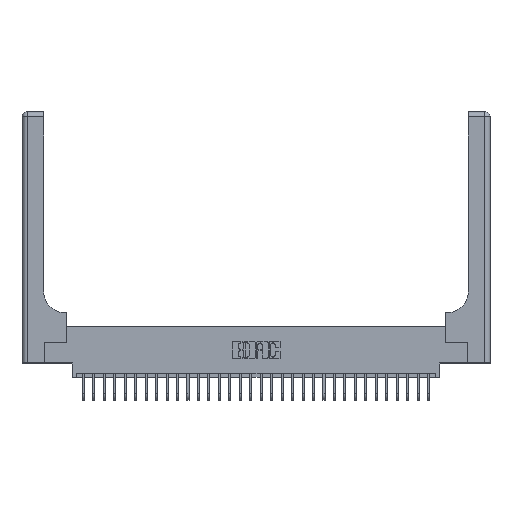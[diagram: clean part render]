
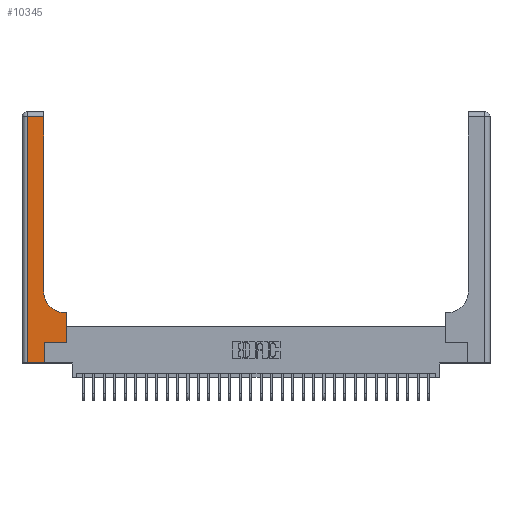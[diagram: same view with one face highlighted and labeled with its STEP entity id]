
A CAD part, top view. The second image highlights one B-rep face of the part: STEP entity #10345.
In plain terms, the highlighted planar face has unit normal (0, 0, 1).
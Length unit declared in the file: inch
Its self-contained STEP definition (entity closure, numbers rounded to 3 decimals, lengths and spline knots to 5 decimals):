
#349 = VECTOR ( 'NONE', #12767, 39.37008 ) ;
#1641 = VERTEX_POINT ( 'NONE', #20341 ) ;
#1968 = EDGE_CURVE ( 'NONE', #17609, #16469, #7856, .T. ) ;
#2002 = CIRCLE ( 'NONE', #9205, 0.25 ) ;
#2087 = LINE ( 'NONE', #19974, #28533 ) ;
#2182 = VERTEX_POINT ( 'NONE', #30388 ) ;
#2671 = LINE ( 'NONE', #3339, #16649 ) ;
#3339 = CARTESIAN_POINT ( 'NONE',  ( 0.265, 0.25, 0.37 ) ) ;
#3849 = VECTOR ( 'NONE', #8884, 39.37008 ) ;
#4074 = CARTESIAN_POINT ( 'NONE',  ( 0.528, 0.6, 0.37 ) ) ;
#4558 = LINE ( 'NONE', #20495, #28813 ) ;
#4676 = VERTEX_POINT ( 'NONE', #22473 ) ;
#5651 = CARTESIAN_POINT ( 'NONE',  ( 0.06, 3., 0.37 ) ) ;
#5925 = ORIENTED_EDGE ( 'NONE', *, *, #27238, .T. ) ;
#6271 = DIRECTION ( 'NONE',  ( -1., 0., 0. ) ) ;
#6275 = LINE ( 'NONE', #26719, #11770 ) ;
#6297 = CARTESIAN_POINT ( 'NONE',  ( 0.06, 2.94, 0.37 ) ) ;
#6916 = LINE ( 'NONE', #16647, #14210 ) ;
#7299 = VERTEX_POINT ( 'NONE', #15905 ) ;
#7306 = AXIS2_PLACEMENT_3D ( 'NONE', #10769, #20183, #6271 ) ;
#7359 = LINE ( 'NONE', #29495, #349 ) ;
#7856 = LINE ( 'NONE', #18640, #3849 ) ;
#8058 = CARTESIAN_POINT ( 'NONE',  ( 0.06, 0., 0.37 ) ) ;
#8654 = DIRECTION ( 'NONE',  ( 0., 1., 0. ) ) ;
#8852 = EDGE_LOOP ( 'NONE', ( #28516, #15959, #13714, #26668, #22316, #29290, #5925, #21931, #28116 ) ) ;
#8884 = DIRECTION ( 'NONE',  ( 1., 0., 0. ) ) ;
#8926 = EDGE_CURVE ( 'NONE', #4676, #24219, #2671, .T. ) ;
#9205 = AXIS2_PLACEMENT_3D ( 'NONE', #27649, #18677, #15988 ) ;
#9849 = VECTOR ( 'NONE', #25295, 39.37008 ) ;
#10345 = ADVANCED_FACE ( 'NONE', ( #15160 ), #22846, .F. ) ;
#10583 = DIRECTION ( 'NONE',  ( 0., 1., 0. ) ) ;
#10769 = CARTESIAN_POINT ( 'NONE',  ( 0., 3., 0.37 ) ) ;
#11770 = VECTOR ( 'NONE', #29083, 39.37008 ) ;
#12767 = DIRECTION ( 'NONE',  ( -1., 0., 0. ) ) ;
#13714 = ORIENTED_EDGE ( 'NONE', *, *, #15154, .T. ) ;
#14210 = VECTOR ( 'NONE', #16455, 39.37008 ) ;
#15139 = DIRECTION ( 'NONE',  ( 1., 0., 0. ) ) ;
#15154 = EDGE_CURVE ( 'NONE', #22289, #17609, #27829, .T. ) ;
#15160 = FACE_OUTER_BOUND ( 'NONE', #8852, .T. ) ;
#15905 = CARTESIAN_POINT ( 'NONE',  ( 0.26, 0.85, 0.37 ) ) ;
#15959 = ORIENTED_EDGE ( 'NONE', *, *, #23742, .T. ) ;
#15988 = DIRECTION ( 'NONE',  ( 1., 0., 0. ) ) ;
#16455 = DIRECTION ( 'NONE',  ( 0., 1., 0. ) ) ;
#16469 = VERTEX_POINT ( 'NONE', #17947 ) ;
#16647 = CARTESIAN_POINT ( 'NONE',  ( 0.528, 0.25, 0.37 ) ) ;
#16649 = VECTOR ( 'NONE', #15139, 39.37008 ) ;
#17053 = EDGE_CURVE ( 'NONE', #2182, #7299, #2002, .T. ) ;
#17589 = EDGE_CURVE ( 'NONE', #23135, #2182, #6275, .T. ) ;
#17609 = VERTEX_POINT ( 'NONE', #8058 ) ;
#17947 = CARTESIAN_POINT ( 'NONE',  ( 0.265, 0., 0.37 ) ) ;
#18640 = CARTESIAN_POINT ( 'NONE',  ( 0., 0., 0.37 ) ) ;
#18677 = DIRECTION ( 'NONE',  ( 0., 0., -1. ) ) ;
#19974 = CARTESIAN_POINT ( 'NONE',  ( 0.265, 0., 0.37 ) ) ;
#20183 = DIRECTION ( 'NONE',  ( 0., 0., -1. ) ) ;
#20341 = CARTESIAN_POINT ( 'NONE',  ( 0.26, 2.94, 0.37 ) ) ;
#20495 = CARTESIAN_POINT ( 'NONE',  ( 0.26, 3., 0.37 ) ) ;
#21931 = ORIENTED_EDGE ( 'NONE', *, *, #17589, .T. ) ;
#22289 = VERTEX_POINT ( 'NONE', #6297 ) ;
#22316 = ORIENTED_EDGE ( 'NONE', *, *, #27543, .T. ) ;
#22473 = CARTESIAN_POINT ( 'NONE',  ( 0.265, 0.25, 0.37 ) ) ;
#22846 = PLANE ( 'NONE',  #7306 ) ;
#23135 = VERTEX_POINT ( 'NONE', #4074 ) ;
#23742 = EDGE_CURVE ( 'NONE', #1641, #22289, #7359, .T. ) ;
#24219 = VERTEX_POINT ( 'NONE', #29044 ) ;
#25295 = DIRECTION ( 'NONE',  ( 0., -1., 0. ) ) ;
#26668 = ORIENTED_EDGE ( 'NONE', *, *, #1968, .T. ) ;
#26719 = CARTESIAN_POINT ( 'NONE',  ( 0.26, 0.6, 0.37 ) ) ;
#27238 = EDGE_CURVE ( 'NONE', #24219, #23135, #6916, .T. ) ;
#27543 = EDGE_CURVE ( 'NONE', #16469, #4676, #2087, .T. ) ;
#27649 = CARTESIAN_POINT ( 'NONE',  ( 0.51, 0.85, 0.37 ) ) ;
#27829 = LINE ( 'NONE', #5651, #9849 ) ;
#28116 = ORIENTED_EDGE ( 'NONE', *, *, #17053, .T. ) ;
#28516 = ORIENTED_EDGE ( 'NONE', *, *, #29607, .T. ) ;
#28533 = VECTOR ( 'NONE', #10583, 39.37008 ) ;
#28813 = VECTOR ( 'NONE', #8654, 39.37008 ) ;
#29044 = CARTESIAN_POINT ( 'NONE',  ( 0.528, 0.25, 0.37 ) ) ;
#29083 = DIRECTION ( 'NONE',  ( -1., 0., 0. ) ) ;
#29290 = ORIENTED_EDGE ( 'NONE', *, *, #8926, .T. ) ;
#29495 = CARTESIAN_POINT ( 'NONE',  ( 0., 2.94, 0.37 ) ) ;
#29607 = EDGE_CURVE ( 'NONE', #7299, #1641, #4558, .T. ) ;
#30388 = CARTESIAN_POINT ( 'NONE',  ( 0.51, 0.6, 0.37 ) ) ;
